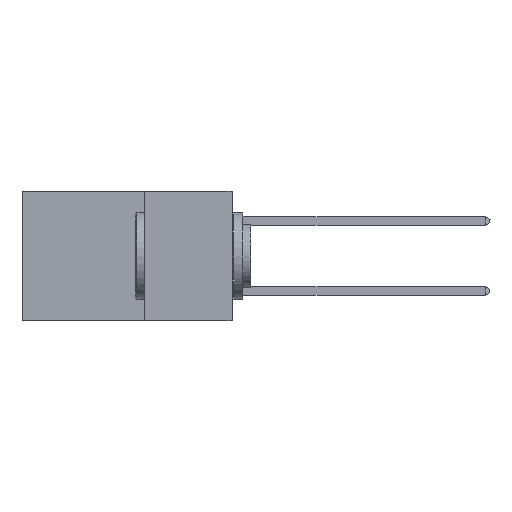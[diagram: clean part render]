
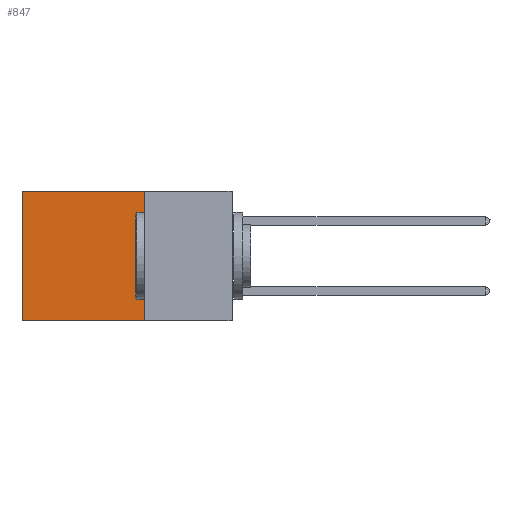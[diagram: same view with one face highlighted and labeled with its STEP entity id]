
A CAD part, left-side view. The second image highlights one B-rep face of the part: STEP entity #847.
In plain terms, the highlighted planar face has unit normal (-1, 0, 0).
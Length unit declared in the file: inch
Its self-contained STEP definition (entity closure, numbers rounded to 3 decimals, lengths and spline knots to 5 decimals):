
#347 = VERTEX_POINT ( 'NONE', #2218 ) ;
#702 = ORIENTED_EDGE ( 'NONE', *, *, #11111, .T. ) ;
#847 = ADVANCED_FACE ( 'NONE', ( #14560 ), #5734, .F. ) ;
#911 = EDGE_CURVE ( 'NONE', #15110, #347, #8046, .T. ) ;
#944 = VECTOR ( 'NONE', #8932, 39.37008 ) ;
#1055 = CARTESIAN_POINT ( 'NONE',  ( 0.2875, 0.25, -0.37 ) ) ;
#1444 = LINE ( 'NONE', #11820, #944 ) ;
#1878 = DIRECTION ( 'NONE',  ( 0., 0., -1. ) ) ;
#2218 = CARTESIAN_POINT ( 'NONE',  ( 0.2875, 0.6, -0.37 ) ) ;
#2584 = CARTESIAN_POINT ( 'NONE',  ( 0.2875, 0.25, 0. ) ) ;
#4203 = DIRECTION ( 'NONE',  ( 0., 0., -1. ) ) ;
#4245 = VECTOR ( 'NONE', #12538, 39.37008 ) ;
#4540 = CARTESIAN_POINT ( 'NONE',  ( 0.2875, 0.25, -0.37 ) ) ;
#5734 = PLANE ( 'NONE',  #8694 ) ;
#7138 = LINE ( 'NONE', #9821, #7385 ) ;
#7311 = VECTOR ( 'NONE', #16993, 39.37008 ) ;
#7385 = VECTOR ( 'NONE', #1878, 39.37008 ) ;
#8046 = LINE ( 'NONE', #1055, #7311 ) ;
#8258 = EDGE_CURVE ( 'NONE', #11683, #15110, #7138, .T. ) ;
#8694 = AXIS2_PLACEMENT_3D ( 'NONE', #2584, #13754, #4203 ) ;
#8932 = DIRECTION ( 'NONE',  ( 0., 0., -1. ) ) ;
#9105 = ORIENTED_EDGE ( 'NONE', *, *, #8258, .F. ) ;
#9821 = CARTESIAN_POINT ( 'NONE',  ( 0.2875, 0.25, 0. ) ) ;
#10428 = CARTESIAN_POINT ( 'NONE',  ( 0.2875, 0.6, 0. ) ) ;
#11111 = EDGE_CURVE ( 'NONE', #18140, #347, #1444, .T. ) ;
#11683 = VERTEX_POINT ( 'NONE', #19739 ) ;
#11820 = CARTESIAN_POINT ( 'NONE',  ( 0.2875, 0.6, 0. ) ) ;
#12538 = DIRECTION ( 'NONE',  ( 0., 1., 0. ) ) ;
#13718 = ORIENTED_EDGE ( 'NONE', *, *, #911, .F. ) ;
#13731 = LINE ( 'NONE', #15792, #4245 ) ;
#13754 = DIRECTION ( 'NONE',  ( 1., 0., 0. ) ) ;
#14560 = FACE_OUTER_BOUND ( 'NONE', #15640, .T. ) ;
#15110 = VERTEX_POINT ( 'NONE', #4540 ) ;
#15640 = EDGE_LOOP ( 'NONE', ( #702, #13718, #9105, #18571 ) ) ;
#15792 = CARTESIAN_POINT ( 'NONE',  ( 0.2875, 0.25, 0. ) ) ;
#16993 = DIRECTION ( 'NONE',  ( 0., 1., 0. ) ) ;
#17187 = EDGE_CURVE ( 'NONE', #11683, #18140, #13731, .T. ) ;
#18140 = VERTEX_POINT ( 'NONE', #10428 ) ;
#18571 = ORIENTED_EDGE ( 'NONE', *, *, #17187, .T. ) ;
#19739 = CARTESIAN_POINT ( 'NONE',  ( 0.2875, 0.25, 0. ) ) ;
